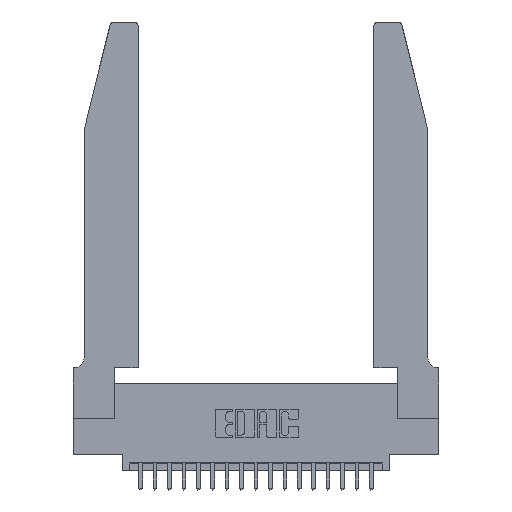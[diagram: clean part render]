
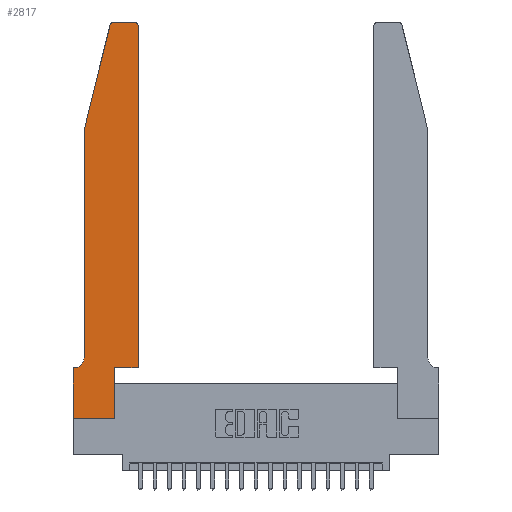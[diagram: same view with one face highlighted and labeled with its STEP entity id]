
A CAD part, top view. The second image highlights one B-rep face of the part: STEP entity #2817.
In plain terms, the highlighted planar face has unit normal (0, 0, 1).
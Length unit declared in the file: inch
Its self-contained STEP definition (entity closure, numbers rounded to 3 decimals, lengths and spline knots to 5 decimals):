
#131 = EDGE_CURVE ( 'NONE', #14970, #4738, #2928, .T. ) ;
#201 = EDGE_CURVE ( 'NONE', #11157, #13033, #13118, .T. ) ;
#662 = CIRCLE ( 'NONE', #10599, 0.03 ) ;
#1102 = CARTESIAN_POINT ( 'NONE',  ( 0.284, 2.72, 0.37 ) ) ;
#1110 = DIRECTION ( 'NONE',  ( 0., -1., 0. ) ) ;
#1245 = ORIENTED_EDGE ( 'NONE', *, *, #9484, .T. ) ;
#1355 = CARTESIAN_POINT ( 'NONE',  ( 0.0755, 2., 0.37 ) ) ;
#1429 = VECTOR ( 'NONE', #18637, 39.37008 ) ;
#1517 = DIRECTION ( 'NONE',  ( 0., 0., 1. ) ) ;
#1593 = CARTESIAN_POINT ( 'NONE',  ( 0.4505, 0.35, 0.37 ) ) ;
#2113 = CARTESIAN_POINT ( 'NONE',  ( 0.25487, 2.72718, 0.37 ) ) ;
#2639 = ORIENTED_EDGE ( 'NONE', *, *, #3441, .T. ) ;
#2787 = DIRECTION ( 'NONE',  ( 0., 0., 1. ) ) ;
#2817 = ADVANCED_FACE ( 'NONE', ( #15889 ), #16404, .T. ) ;
#2820 = DIRECTION ( 'NONE',  ( -0.239, -0.971, 0. ) ) ;
#2928 = CIRCLE ( 'NONE', #6948, 0.07 ) ;
#2950 = DIRECTION ( 'NONE',  ( 0., 0., 1. ) ) ;
#3441 = EDGE_CURVE ( 'NONE', #11460, #14016, #4615, .T. ) ;
#3616 = EDGE_CURVE ( 'NONE', #14016, #10175, #662, .T. ) ;
#3704 = VECTOR ( 'NONE', #8721, 39.37008 ) ;
#4228 = VECTOR ( 'NONE', #16540, 39.37008 ) ;
#4369 = CARTESIAN_POINT ( 'NONE',  ( 0.284, 2.75, 0.37 ) ) ;
#4444 = EDGE_CURVE ( 'NONE', #10540, #16018, #21524, .T. ) ;
#4615 = LINE ( 'NONE', #21382, #11949 ) ;
#4738 = VERTEX_POINT ( 'NONE', #18426 ) ;
#5333 = EDGE_CURVE ( 'NONE', #20856, #14970, #17638, .T. ) ;
#5385 = CARTESIAN_POINT ( 'NONE',  ( 0.2865, 0.35, 0.37 ) ) ;
#5943 = DIRECTION ( 'NONE',  ( 1., 0., 0. ) ) ;
#6753 = LINE ( 'NONE', #5385, #12510 ) ;
#6948 = AXIS2_PLACEMENT_3D ( 'NONE', #16061, #7992, #16645 ) ;
#7148 = VERTEX_POINT ( 'NONE', #15126 ) ;
#7149 = LINE ( 'NONE', #16990, #9502 ) ;
#7232 = CARTESIAN_POINT ( 'NONE',  ( 0.0755, 0.42, 0.37 ) ) ;
#7245 = ORIENTED_EDGE ( 'NONE', *, *, #10266, .T. ) ;
#7306 = EDGE_CURVE ( 'NONE', #7148, #11157, #19898, .T. ) ;
#7992 = DIRECTION ( 'NONE',  ( 0., 0., -1. ) ) ;
#8022 = DIRECTION ( 'NONE',  ( 1., 0., 0. ) ) ;
#8124 = CARTESIAN_POINT ( 'NONE',  ( 0., 0.35, 0.37 ) ) ;
#8556 = ORIENTED_EDGE ( 'NONE', *, *, #7306, .T. ) ;
#8721 = DIRECTION ( 'NONE',  ( 0., -1., 0. ) ) ;
#8873 = VECTOR ( 'NONE', #9112, 39.37008 ) ;
#9053 = ORIENTED_EDGE ( 'NONE', *, *, #20512, .T. ) ;
#9112 = DIRECTION ( 'NONE',  ( 1., 0., 0. ) ) ;
#9484 = EDGE_CURVE ( 'NONE', #16018, #11460, #20882, .T. ) ;
#9502 = VECTOR ( 'NONE', #2820, 39.37008 ) ;
#10038 = DIRECTION ( 'NONE',  ( -1., 0., 0. ) ) ;
#10175 = VERTEX_POINT ( 'NONE', #2113 ) ;
#10266 = EDGE_CURVE ( 'NONE', #21462, #10540, #10410, .T. ) ;
#10410 = LINE ( 'NONE', #14598, #8873 ) ;
#10437 = DIRECTION ( 'NONE',  ( 0., 1., 0. ) ) ;
#10526 = AXIS2_PLACEMENT_3D ( 'NONE', #18114, #2950, #8022 ) ;
#10540 = VERTEX_POINT ( 'NONE', #1593 ) ;
#10599 = AXIS2_PLACEMENT_3D ( 'NONE', #1102, #2787, #5943 ) ;
#11157 = VERTEX_POINT ( 'NONE', #19027 ) ;
#11221 = CARTESIAN_POINT ( 'NONE',  ( 0.2865, 0.35, 0.37 ) ) ;
#11338 = ORIENTED_EDGE ( 'NONE', *, *, #13979, .T. ) ;
#11460 = VERTEX_POINT ( 'NONE', #18797 ) ;
#11639 = DIRECTION ( 'NONE',  ( -1., 0., 0. ) ) ;
#11949 = VECTOR ( 'NONE', #10038, 39.37008 ) ;
#11977 = CARTESIAN_POINT ( 'NONE',  ( 0.4505, 0.35, 0.37 ) ) ;
#12254 = LINE ( 'NONE', #14986, #19808 ) ;
#12510 = VECTOR ( 'NONE', #10437, 39.37008 ) ;
#12545 = CARTESIAN_POINT ( 'NONE',  ( 0.0755, 2., 0.37 ) ) ;
#13033 = VERTEX_POINT ( 'NONE', #19941 ) ;
#13118 = LINE ( 'NONE', #16616, #4228 ) ;
#13266 = AXIS2_PLACEMENT_3D ( 'NONE', #8124, #1517, #16971 ) ;
#13979 = EDGE_CURVE ( 'NONE', #10175, #20856, #7149, .T. ) ;
#14016 = VERTEX_POINT ( 'NONE', #4369 ) ;
#14203 = EDGE_LOOP ( 'NONE', ( #2639, #16016, #11338, #15484, #16170, #15557, #8556, #21568, #9053, #7245, #17347, #1245 ) ) ;
#14542 = VECTOR ( 'NONE', #1110, 39.37008 ) ;
#14598 = CARTESIAN_POINT ( 'NONE',  ( 0.4505, 0.35, 0.37 ) ) ;
#14970 = VERTEX_POINT ( 'NONE', #7232 ) ;
#14986 = CARTESIAN_POINT ( 'NONE',  ( 0.0755, 0.35, 0.37 ) ) ;
#15126 = CARTESIAN_POINT ( 'NONE',  ( 0., 0.35, 0.37 ) ) ;
#15484 = ORIENTED_EDGE ( 'NONE', *, *, #5333, .T. ) ;
#15557 = ORIENTED_EDGE ( 'NONE', *, *, #20305, .T. ) ;
#15889 = FACE_OUTER_BOUND ( 'NONE', #14203, .T. ) ;
#16016 = ORIENTED_EDGE ( 'NONE', *, *, #3616, .T. ) ;
#16018 = VERTEX_POINT ( 'NONE', #19851 ) ;
#16061 = CARTESIAN_POINT ( 'NONE',  ( 0.0055, 0.42, 0.37 ) ) ;
#16170 = ORIENTED_EDGE ( 'NONE', *, *, #131, .T. ) ;
#16404 = PLANE ( 'NONE',  #13266 ) ;
#16540 = DIRECTION ( 'NONE',  ( 1., 0., 0. ) ) ;
#16616 = CARTESIAN_POINT ( 'NONE',  ( 0., 0., 0.37 ) ) ;
#16645 = DIRECTION ( 'NONE',  ( -1., 0., 0. ) ) ;
#16971 = DIRECTION ( 'NONE',  ( 1., 0., 0. ) ) ;
#16990 = CARTESIAN_POINT ( 'NONE',  ( 0.0755, 2., 0.37 ) ) ;
#17347 = ORIENTED_EDGE ( 'NONE', *, *, #4444, .T. ) ;
#17638 = LINE ( 'NONE', #12545, #14542 ) ;
#18114 = CARTESIAN_POINT ( 'NONE',  ( 0.4205, 2.72, 0.37 ) ) ;
#18426 = CARTESIAN_POINT ( 'NONE',  ( 0.0055, 0.35, 0.37 ) ) ;
#18637 = DIRECTION ( 'NONE',  ( 0., 1., 0. ) ) ;
#18797 = CARTESIAN_POINT ( 'NONE',  ( 0.4205, 2.75, 0.37 ) ) ;
#19027 = CARTESIAN_POINT ( 'NONE',  ( 0., 0., 0.37 ) ) ;
#19808 = VECTOR ( 'NONE', #11639, 39.37008 ) ;
#19851 = CARTESIAN_POINT ( 'NONE',  ( 0.4505, 2.72, 0.37 ) ) ;
#19898 = LINE ( 'NONE', #20492, #3704 ) ;
#19941 = CARTESIAN_POINT ( 'NONE',  ( 0.2865, 0., 0.37 ) ) ;
#20305 = EDGE_CURVE ( 'NONE', #4738, #7148, #12254, .T. ) ;
#20492 = CARTESIAN_POINT ( 'NONE',  ( 0., 0., 0.37 ) ) ;
#20512 = EDGE_CURVE ( 'NONE', #13033, #21462, #6753, .T. ) ;
#20856 = VERTEX_POINT ( 'NONE', #1355 ) ;
#20882 = CIRCLE ( 'NONE', #10526, 0.03 ) ;
#21382 = CARTESIAN_POINT ( 'NONE',  ( 0.2605, 2.75, 0.37 ) ) ;
#21462 = VERTEX_POINT ( 'NONE', #11221 ) ;
#21524 = LINE ( 'NONE', #11977, #1429 ) ;
#21568 = ORIENTED_EDGE ( 'NONE', *, *, #201, .T. ) ;
